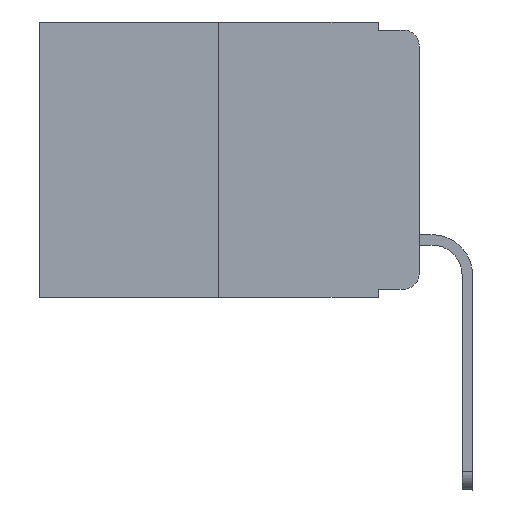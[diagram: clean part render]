
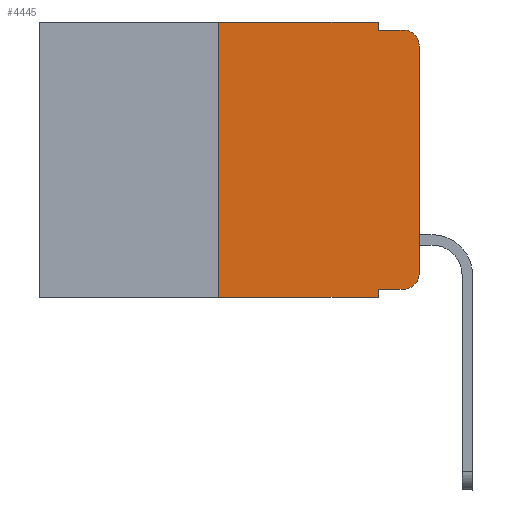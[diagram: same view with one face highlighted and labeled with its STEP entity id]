
A CAD part, left-side view. The second image highlights one B-rep face of the part: STEP entity #4445.
In plain terms, the highlighted planar face has unit normal (-1, 0, 0).
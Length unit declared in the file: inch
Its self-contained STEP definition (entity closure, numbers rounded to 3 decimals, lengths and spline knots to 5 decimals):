
#423 = EDGE_CURVE ( 'NONE', #1832, #14573, #7594, .T. ) ;
#513 = CARTESIAN_POINT ( 'NONE',  ( 0., 0.473, -0.343 ) ) ;
#633 = CARTESIAN_POINT ( 'NONE',  ( 0., 0.473, 0. ) ) ;
#1012 = VERTEX_POINT ( 'NONE', #8745 ) ;
#1127 = ORIENTED_EDGE ( 'NONE', *, *, #8951, .T. ) ;
#1549 = EDGE_CURVE ( 'NONE', #17382, #2435, #7781, .T. ) ;
#1832 = VERTEX_POINT ( 'NONE', #3420 ) ;
#2435 = VERTEX_POINT ( 'NONE', #11786 ) ;
#2814 = CARTESIAN_POINT ( 'NONE',  ( 0., 0., -0.03 ) ) ;
#3230 = LINE ( 'NONE', #513, #15677 ) ;
#3299 = AXIS2_PLACEMENT_3D ( 'NONE', #633, #8863, #4523 ) ;
#3420 = CARTESIAN_POINT ( 'NONE',  ( 0., 0.02, -0.333 ) ) ;
#3663 = CARTESIAN_POINT ( 'NONE',  ( 0., 0.051, 0. ) ) ;
#3879 = VECTOR ( 'NONE', #6756, 39.37008 ) ;
#3955 = VERTEX_POINT ( 'NONE', #10103 ) ;
#3994 = DIRECTION ( 'NONE',  ( 0., 0., -1. ) ) ;
#4040 = EDGE_CURVE ( 'NONE', #1012, #6747, #11764, .T. ) ;
#4116 = ORIENTED_EDGE ( 'NONE', *, *, #4040, .F. ) ;
#4445 = ADVANCED_FACE ( 'NONE', ( #12639 ), #11218, .F. ) ;
#4471 = AXIS2_PLACEMENT_3D ( 'NONE', #16078, #17309, #14669 ) ;
#4523 = DIRECTION ( 'NONE',  ( 0., 0., -1. ) ) ;
#4529 = CARTESIAN_POINT ( 'NONE',  ( 0., 0.051, -0.333 ) ) ;
#4937 = CARTESIAN_POINT ( 'NONE',  ( 0., 0.051, 0. ) ) ;
#5586 = DIRECTION ( 'NONE',  ( 0., -1., 0. ) ) ;
#5751 = VECTOR ( 'NONE', #14927, 39.37008 ) ;
#5870 = ORIENTED_EDGE ( 'NONE', *, *, #13495, .F. ) ;
#5913 = DIRECTION ( 'NONE',  ( 0., -1., 0. ) ) ;
#6195 = VERTEX_POINT ( 'NONE', #2814 ) ;
#6668 = VECTOR ( 'NONE', #17113, 39.37008 ) ;
#6747 = VERTEX_POINT ( 'NONE', #3663 ) ;
#6756 = DIRECTION ( 'NONE',  ( 0., 0., 1. ) ) ;
#7198 = AXIS2_PLACEMENT_3D ( 'NONE', #11562, #15624, #16959 ) ;
#7594 = CIRCLE ( 'NONE', #4471, 0.02 ) ;
#7781 = LINE ( 'NONE', #17387, #10206 ) ;
#7972 = EDGE_CURVE ( 'NONE', #13069, #8569, #3230, .T. ) ;
#8569 = VERTEX_POINT ( 'NONE', #14837 ) ;
#8745 = CARTESIAN_POINT ( 'NONE',  ( 0., 0.25, 0. ) ) ;
#8863 = DIRECTION ( 'NONE',  ( 1., 0., 0. ) ) ;
#8951 = EDGE_CURVE ( 'NONE', #6195, #2435, #13116, .T. ) ;
#9321 = EDGE_CURVE ( 'NONE', #6747, #17382, #11539, .T. ) ;
#9556 = LINE ( 'NONE', #10946, #5751 ) ;
#10078 = EDGE_LOOP ( 'NONE', ( #11541, #1127, #12133, #13160, #4116, #5870, #16029, #15908, #16596, #12874 ) ) ;
#10103 = CARTESIAN_POINT ( 'NONE',  ( 0., 0.051, -0.333 ) ) ;
#10206 = VECTOR ( 'NONE', #16071, 39.37008 ) ;
#10946 = CARTESIAN_POINT ( 'NONE',  ( 0., 0.25, 0. ) ) ;
#11218 = PLANE ( 'NONE',  #3299 ) ;
#11445 = EDGE_CURVE ( 'NONE', #3955, #8569, #11598, .T. ) ;
#11495 = EDGE_CURVE ( 'NONE', #14573, #6195, #13189, .T. ) ;
#11539 = LINE ( 'NONE', #4937, #6668 ) ;
#11541 = ORIENTED_EDGE ( 'NONE', *, *, #11495, .T. ) ;
#11562 = CARTESIAN_POINT ( 'NONE',  ( 0., 0.02, -0.03 ) ) ;
#11598 = LINE ( 'NONE', #16014, #14591 ) ;
#11619 = EDGE_CURVE ( 'NONE', #3955, #1832, #13685, .T. ) ;
#11764 = LINE ( 'NONE', #17165, #14983 ) ;
#11772 = CARTESIAN_POINT ( 'NONE',  ( 0., 0., 0. ) ) ;
#11786 = CARTESIAN_POINT ( 'NONE',  ( 0., 0.02, -0.01 ) ) ;
#12092 = CARTESIAN_POINT ( 'NONE',  ( 0., 0.051, -0.01 ) ) ;
#12133 = ORIENTED_EDGE ( 'NONE', *, *, #1549, .F. ) ;
#12543 = CARTESIAN_POINT ( 'NONE',  ( 0., 0., -0.313 ) ) ;
#12639 = FACE_OUTER_BOUND ( 'NONE', #10078, .T. ) ;
#12874 = ORIENTED_EDGE ( 'NONE', *, *, #423, .T. ) ;
#12910 = CARTESIAN_POINT ( 'NONE',  ( 0., 0.25, -0.343 ) ) ;
#13069 = VERTEX_POINT ( 'NONE', #12910 ) ;
#13116 = CIRCLE ( 'NONE', #7198, 0.02 ) ;
#13160 = ORIENTED_EDGE ( 'NONE', *, *, #9321, .F. ) ;
#13189 = LINE ( 'NONE', #11772, #3879 ) ;
#13495 = EDGE_CURVE ( 'NONE', #13069, #1012, #9556, .T. ) ;
#13685 = LINE ( 'NONE', #4529, #16000 ) ;
#14494 = DIRECTION ( 'NONE',  ( 0., -1., 0. ) ) ;
#14573 = VERTEX_POINT ( 'NONE', #12543 ) ;
#14591 = VECTOR ( 'NONE', #3994, 39.37008 ) ;
#14669 = DIRECTION ( 'NONE',  ( 0., 0., -1. ) ) ;
#14837 = CARTESIAN_POINT ( 'NONE',  ( 0., 0.051, -0.343 ) ) ;
#14927 = DIRECTION ( 'NONE',  ( 0., 0., 1. ) ) ;
#14983 = VECTOR ( 'NONE', #14494, 39.37008 ) ;
#15624 = DIRECTION ( 'NONE',  ( -1., 0., 0. ) ) ;
#15677 = VECTOR ( 'NONE', #5913, 39.37008 ) ;
#15908 = ORIENTED_EDGE ( 'NONE', *, *, #11445, .F. ) ;
#16000 = VECTOR ( 'NONE', #5586, 39.37008 ) ;
#16014 = CARTESIAN_POINT ( 'NONE',  ( 0., 0.051, 0. ) ) ;
#16029 = ORIENTED_EDGE ( 'NONE', *, *, #7972, .T. ) ;
#16071 = DIRECTION ( 'NONE',  ( 0., -1., 0. ) ) ;
#16078 = CARTESIAN_POINT ( 'NONE',  ( 0., 0.02, -0.313 ) ) ;
#16596 = ORIENTED_EDGE ( 'NONE', *, *, #11619, .T. ) ;
#16959 = DIRECTION ( 'NONE',  ( 0., 0., -1. ) ) ;
#17113 = DIRECTION ( 'NONE',  ( 0., 0., -1. ) ) ;
#17165 = CARTESIAN_POINT ( 'NONE',  ( 0., 0.473, 0. ) ) ;
#17309 = DIRECTION ( 'NONE',  ( -1., 0., 0. ) ) ;
#17382 = VERTEX_POINT ( 'NONE', #12092 ) ;
#17387 = CARTESIAN_POINT ( 'NONE',  ( 0., 0.051, -0.01 ) ) ;
